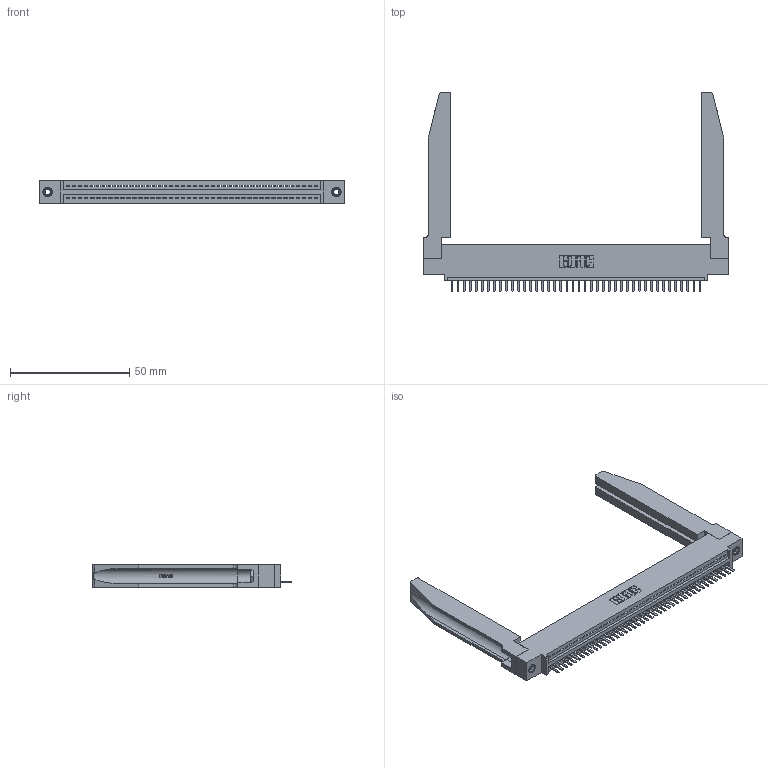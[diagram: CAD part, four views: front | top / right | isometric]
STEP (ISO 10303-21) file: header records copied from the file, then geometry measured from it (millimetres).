
FILE_DESCRIPTION (( 'STEP AP203' ), '1' );
FILE_NAME ('345-042-520-478.STEP', '2019-10-08T13:42:03', ( '' ), ( '' ), 'SwSTEP 2.0', 'SolidWorks 2016', '' );
FILE_SCHEMA (( 'CONFIG_CONTROL_DESIGN' ));
Length unit declared in the file: inch
Products named in the file (5): 345-220-078_345-220-078; 345-292-001_345-293-120; 345-042-520-478; 345-250-001_345-250-001-102; 345 Part_0.110 Offset - 0.156 Dia-TH
Assembly tree (47 placements, depth 2):
  345-042-520-478
    345 Part_0.110 Offset - 0.156 Dia-TH
    345-292-001_345-293-120  x42
    345-250-001_345-250-001-102  x2
    345-220-078_345-220-078  x2
Bounding box: 127.91 x 83.44 x 9.4 mm (x, y, z)
Volume: 19725.7 mm3; surface area: 22419.7 mm2
Topology: 47 solids, 47 shells, 2968 faces, 8689 edges, 5670 vertices
Faces by surface type: plane 1990, cylinder 926, bspline 36, cone 12, torus 4
Entity records: 36596 total; most frequent: CARTESIAN_POINT 7249, ORIENTED_EDGE 6110, DIRECTION 5325, EDGE_CURVE 3055, LINE 2657, VECTOR 2657, VERTEX_POINT 2028, AXIS2_PLACEMENT_3D 1334
